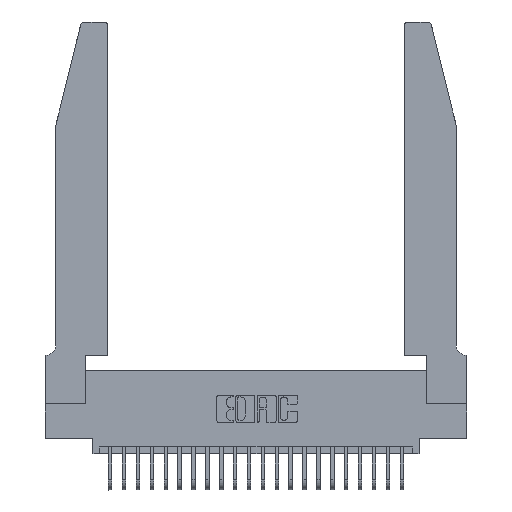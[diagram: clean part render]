
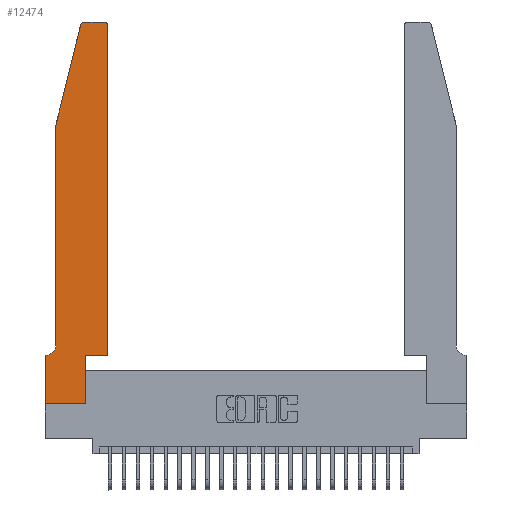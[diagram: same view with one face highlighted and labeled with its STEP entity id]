
A CAD part, top view. The second image highlights one B-rep face of the part: STEP entity #12474.
In plain terms, the highlighted planar face has unit normal (0, 0, 1).
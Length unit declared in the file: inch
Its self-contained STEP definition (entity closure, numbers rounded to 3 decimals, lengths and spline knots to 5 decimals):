
#636 = ORIENTED_EDGE ( 'NONE', *, *, #8559, .T. ) ;
#1060 = LINE ( 'NONE', #9096, #5590 ) ;
#1233 = PLANE ( 'NONE',  #10014 ) ;
#1410 = ORIENTED_EDGE ( 'NONE', *, *, #19503, .T. ) ;
#1574 = DIRECTION ( 'NONE',  ( 1., 0., 0. ) ) ;
#1803 = CARTESIAN_POINT ( 'NONE',  ( 0.0755, 2., 0.37 ) ) ;
#2240 = CARTESIAN_POINT ( 'NONE',  ( 0.0755, 0.42, 0.37 ) ) ;
#2585 = VERTEX_POINT ( 'NONE', #14243 ) ;
#2618 = ORIENTED_EDGE ( 'NONE', *, *, #21266, .T. ) ;
#2663 = VECTOR ( 'NONE', #10216, 39.37008 ) ;
#2725 = VECTOR ( 'NONE', #18465, 39.37008 ) ;
#3078 = CARTESIAN_POINT ( 'NONE',  ( 0.2605, 2.75, 0.37 ) ) ;
#3369 = CARTESIAN_POINT ( 'NONE',  ( 0.0755, 2., 0.37 ) ) ;
#3852 = CARTESIAN_POINT ( 'NONE',  ( 0.4205, 2.72, 0.37 ) ) ;
#4040 = EDGE_CURVE ( 'NONE', #2585, #13156, #10618, .T. ) ;
#4077 = CARTESIAN_POINT ( 'NONE',  ( 0.284, 2.75, 0.37 ) ) ;
#4519 = VERTEX_POINT ( 'NONE', #20174 ) ;
#4852 = LINE ( 'NONE', #19220, #23373 ) ;
#4989 = DIRECTION ( 'NONE',  ( -1., 0., 0. ) ) ;
#5033 = ORIENTED_EDGE ( 'NONE', *, *, #13239, .T. ) ;
#5052 = CARTESIAN_POINT ( 'NONE',  ( 0.0755, 0.35, 0.37 ) ) ;
#5147 = DIRECTION ( 'NONE',  ( 1., 0., 0. ) ) ;
#5254 = DIRECTION ( 'NONE',  ( -0.239, -0.971, 0. ) ) ;
#5590 = VECTOR ( 'NONE', #1574, 39.37008 ) ;
#5714 = DIRECTION ( 'NONE',  ( 1., 0., 0. ) ) ;
#5859 = VECTOR ( 'NONE', #6901, 39.37008 ) ;
#6129 = ORIENTED_EDGE ( 'NONE', *, *, #18517, .T. ) ;
#6649 = VERTEX_POINT ( 'NONE', #17819 ) ;
#6667 = AXIS2_PLACEMENT_3D ( 'NONE', #3852, #16829, #5714 ) ;
#6747 = VERTEX_POINT ( 'NONE', #16286 ) ;
#6761 = CARTESIAN_POINT ( 'NONE',  ( 0.284, 2.72, 0.37 ) ) ;
#6901 = DIRECTION ( 'NONE',  ( -1., 0., 0. ) ) ;
#7155 = CIRCLE ( 'NONE', #17790, 0.07 ) ;
#7444 = DIRECTION ( 'NONE',  ( 0., -1., 0. ) ) ;
#8266 = LINE ( 'NONE', #8368, #2663 ) ;
#8368 = CARTESIAN_POINT ( 'NONE',  ( 0., 0., 0.37 ) ) ;
#8559 = EDGE_CURVE ( 'NONE', #20934, #4519, #12724, .T. ) ;
#8645 = DIRECTION ( 'NONE',  ( 1., 0., 0. ) ) ;
#9080 = CARTESIAN_POINT ( 'NONE',  ( 0.0055, 0.42, 0.37 ) ) ;
#9096 = CARTESIAN_POINT ( 'NONE',  ( 0.4505, 0.35, 0.37 ) ) ;
#9148 = CARTESIAN_POINT ( 'NONE',  ( 0.4505, 0.35, 0.37 ) ) ;
#9290 = EDGE_CURVE ( 'NONE', #16012, #21690, #16296, .T. ) ;
#9892 = DIRECTION ( 'NONE',  ( 0., -1., 0. ) ) ;
#10014 = AXIS2_PLACEMENT_3D ( 'NONE', #14381, #16231, #5147 ) ;
#10143 = AXIS2_PLACEMENT_3D ( 'NONE', #6761, #19742, #8645 ) ;
#10216 = DIRECTION ( 'NONE',  ( 1., 0., 0. ) ) ;
#10472 = ORIENTED_EDGE ( 'NONE', *, *, #21864, .T. ) ;
#10618 = CIRCLE ( 'NONE', #6667, 0.03 ) ;
#10640 = ORIENTED_EDGE ( 'NONE', *, *, #23883, .T. ) ;
#10801 = VERTEX_POINT ( 'NONE', #18858 ) ;
#10945 = DIRECTION ( 'NONE',  ( -1., 0., 0. ) ) ;
#11133 = EDGE_CURVE ( 'NONE', #13156, #20934, #14803, .T. ) ;
#12306 = CARTESIAN_POINT ( 'NONE',  ( 0.2865, 0., 0.37 ) ) ;
#12376 = LINE ( 'NONE', #3369, #16140 ) ;
#12474 = ADVANCED_FACE ( 'NONE', ( #19077 ), #1233, .T. ) ;
#12724 = CIRCLE ( 'NONE', #10143, 0.03 ) ;
#12932 = EDGE_LOOP ( 'NONE', ( #15287, #636, #6129, #23774, #10640, #20256, #17552, #1410, #5033, #2618, #10472, #20871 ) ) ;
#13156 = VERTEX_POINT ( 'NONE', #18071 ) ;
#13239 = EDGE_CURVE ( 'NONE', #13576, #6747, #17585, .T. ) ;
#13576 = VERTEX_POINT ( 'NONE', #12306 ) ;
#13920 = CARTESIAN_POINT ( 'NONE',  ( 0., 0., 0.37 ) ) ;
#14243 = CARTESIAN_POINT ( 'NONE',  ( 0.4505, 2.72, 0.37 ) ) ;
#14381 = CARTESIAN_POINT ( 'NONE',  ( 0., 0.35, 0.37 ) ) ;
#14803 = LINE ( 'NONE', #3078, #24038 ) ;
#15069 = EDGE_CURVE ( 'NONE', #6649, #19986, #17494, .T. ) ;
#15287 = ORIENTED_EDGE ( 'NONE', *, *, #11133, .T. ) ;
#16012 = VERTEX_POINT ( 'NONE', #21013 ) ;
#16140 = VECTOR ( 'NONE', #5254, 39.37008 ) ;
#16231 = DIRECTION ( 'NONE',  ( 0., 0., 1. ) ) ;
#16286 = CARTESIAN_POINT ( 'NONE',  ( 0.2865, 0.35, 0.37 ) ) ;
#16296 = LINE ( 'NONE', #5052, #5859 ) ;
#16604 = CARTESIAN_POINT ( 'NONE',  ( 0.2865, 0.35, 0.37 ) ) ;
#16829 = DIRECTION ( 'NONE',  ( 0., 0., 1. ) ) ;
#16835 = LINE ( 'NONE', #9148, #21156 ) ;
#17494 = LINE ( 'NONE', #1803, #18080 ) ;
#17552 = ORIENTED_EDGE ( 'NONE', *, *, #23569, .T. ) ;
#17585 = LINE ( 'NONE', #16604, #2725 ) ;
#17790 = AXIS2_PLACEMENT_3D ( 'NONE', #9080, #22020, #10945 ) ;
#17819 = CARTESIAN_POINT ( 'NONE',  ( 0.0755, 2., 0.37 ) ) ;
#18071 = CARTESIAN_POINT ( 'NONE',  ( 0.4205, 2.75, 0.37 ) ) ;
#18080 = VECTOR ( 'NONE', #7444, 39.37008 ) ;
#18465 = DIRECTION ( 'NONE',  ( 0., 1., 0. ) ) ;
#18517 = EDGE_CURVE ( 'NONE', #4519, #6649, #12376, .T. ) ;
#18858 = CARTESIAN_POINT ( 'NONE',  ( 0.4505, 0.35, 0.37 ) ) ;
#18922 = VERTEX_POINT ( 'NONE', #13920 ) ;
#19077 = FACE_OUTER_BOUND ( 'NONE', #12932, .T. ) ;
#19220 = CARTESIAN_POINT ( 'NONE',  ( 0., 0., 0.37 ) ) ;
#19503 = EDGE_CURVE ( 'NONE', #18922, #13576, #8266, .T. ) ;
#19742 = DIRECTION ( 'NONE',  ( 0., 0., 1. ) ) ;
#19986 = VERTEX_POINT ( 'NONE', #2240 ) ;
#20174 = CARTESIAN_POINT ( 'NONE',  ( 0.25487, 2.72718, 0.37 ) ) ;
#20224 = DIRECTION ( 'NONE',  ( 0., 1., 0. ) ) ;
#20256 = ORIENTED_EDGE ( 'NONE', *, *, #9290, .T. ) ;
#20871 = ORIENTED_EDGE ( 'NONE', *, *, #4040, .T. ) ;
#20934 = VERTEX_POINT ( 'NONE', #4077 ) ;
#21013 = CARTESIAN_POINT ( 'NONE',  ( 0.0055, 0.35, 0.37 ) ) ;
#21156 = VECTOR ( 'NONE', #20224, 39.37008 ) ;
#21266 = EDGE_CURVE ( 'NONE', #6747, #10801, #1060, .T. ) ;
#21690 = VERTEX_POINT ( 'NONE', #23472 ) ;
#21864 = EDGE_CURVE ( 'NONE', #10801, #2585, #16835, .T. ) ;
#22020 = DIRECTION ( 'NONE',  ( 0., 0., -1. ) ) ;
#23373 = VECTOR ( 'NONE', #9892, 39.37008 ) ;
#23472 = CARTESIAN_POINT ( 'NONE',  ( 0., 0.35, 0.37 ) ) ;
#23569 = EDGE_CURVE ( 'NONE', #21690, #18922, #4852, .T. ) ;
#23774 = ORIENTED_EDGE ( 'NONE', *, *, #15069, .T. ) ;
#23883 = EDGE_CURVE ( 'NONE', #19986, #16012, #7155, .T. ) ;
#24038 = VECTOR ( 'NONE', #4989, 39.37008 ) ;
